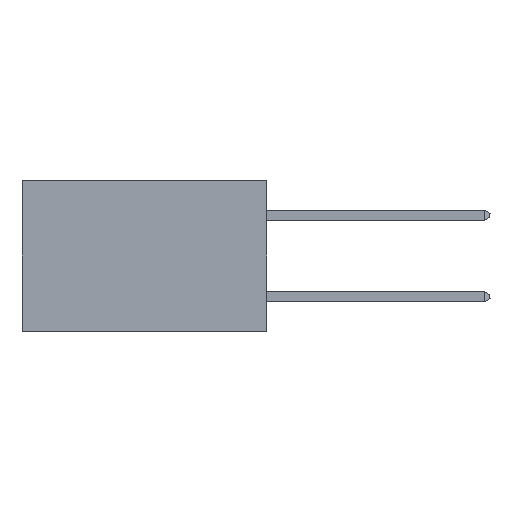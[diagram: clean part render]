
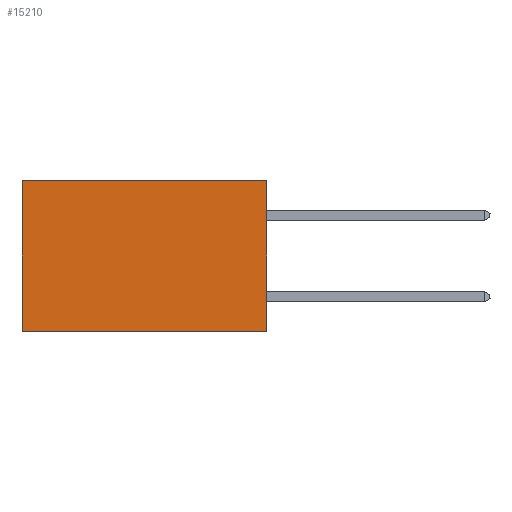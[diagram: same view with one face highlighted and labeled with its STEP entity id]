
A CAD part, left-side view. The second image highlights one B-rep face of the part: STEP entity #15210.
In plain terms, the highlighted planar face has unit normal (-1, 0, 0).
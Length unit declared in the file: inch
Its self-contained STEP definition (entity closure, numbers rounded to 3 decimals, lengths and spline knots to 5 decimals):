
#272 = CARTESIAN_POINT ( 'NONE',  ( 0.2875, 0., 0. ) ) ;
#471 = DIRECTION ( 'NONE',  ( 1., 0., 0. ) ) ;
#830 = DIRECTION ( 'NONE',  ( 0., 1., 0. ) ) ;
#911 = EDGE_CURVE ( 'NONE', #12627, #9120, #11523, .T. ) ;
#1150 = EDGE_LOOP ( 'NONE', ( #9916, #14616, #4330, #1160 ) ) ;
#1160 = ORIENTED_EDGE ( 'NONE', *, *, #911, .T. ) ;
#2102 = CARTESIAN_POINT ( 'NONE',  ( 0.2875, 0., 0. ) ) ;
#2322 = CARTESIAN_POINT ( 'NONE',  ( 0.2875, 0.6, 0. ) ) ;
#2862 = DIRECTION ( 'NONE',  ( 0., 1., 0. ) ) ;
#2895 = DIRECTION ( 'NONE',  ( 0., 0., -1. ) ) ;
#3319 = VECTOR ( 'NONE', #830, 39.37008 ) ;
#4330 = ORIENTED_EDGE ( 'NONE', *, *, #5198, .F. ) ;
#4775 = CARTESIAN_POINT ( 'NONE',  ( 0.2875, 0.6, -0.37 ) ) ;
#5198 = EDGE_CURVE ( 'NONE', #12627, #6310, #13121, .T. ) ;
#5788 = DIRECTION ( 'NONE',  ( 0., 0., -1. ) ) ;
#6203 = FACE_OUTER_BOUND ( 'NONE', #1150, .T. ) ;
#6310 = VERTEX_POINT ( 'NONE', #11401 ) ;
#6356 = PLANE ( 'NONE',  #12276 ) ;
#8015 = CARTESIAN_POINT ( 'NONE',  ( 0.2875, 0., 0. ) ) ;
#8324 = LINE ( 'NONE', #11435, #10438 ) ;
#9120 = VERTEX_POINT ( 'NONE', #2322 ) ;
#9150 = VERTEX_POINT ( 'NONE', #4775 ) ;
#9284 = CARTESIAN_POINT ( 'NONE',  ( 0.2875, 0., 0. ) ) ;
#9679 = EDGE_CURVE ( 'NONE', #9120, #9150, #13196, .T. ) ;
#9916 = ORIENTED_EDGE ( 'NONE', *, *, #9679, .T. ) ;
#10438 = VECTOR ( 'NONE', #2862, 39.37008 ) ;
#10882 = DIRECTION ( 'NONE',  ( 0., 0., -1. ) ) ;
#11401 = CARTESIAN_POINT ( 'NONE',  ( 0.2875, 0., -0.37 ) ) ;
#11435 = CARTESIAN_POINT ( 'NONE',  ( 0.2875, 0., -0.37 ) ) ;
#11523 = LINE ( 'NONE', #9284, #3319 ) ;
#12050 = VECTOR ( 'NONE', #10882, 39.37008 ) ;
#12234 = CARTESIAN_POINT ( 'NONE',  ( 0.2875, 0.6, 0. ) ) ;
#12276 = AXIS2_PLACEMENT_3D ( 'NONE', #272, #471, #2895 ) ;
#12627 = VERTEX_POINT ( 'NONE', #2102 ) ;
#13121 = LINE ( 'NONE', #8015, #15502 ) ;
#13196 = LINE ( 'NONE', #12234, #12050 ) ;
#14220 = EDGE_CURVE ( 'NONE', #6310, #9150, #8324, .T. ) ;
#14616 = ORIENTED_EDGE ( 'NONE', *, *, #14220, .F. ) ;
#15210 = ADVANCED_FACE ( 'NONE', ( #6203 ), #6356, .F. ) ;
#15502 = VECTOR ( 'NONE', #5788, 39.37008 ) ;
